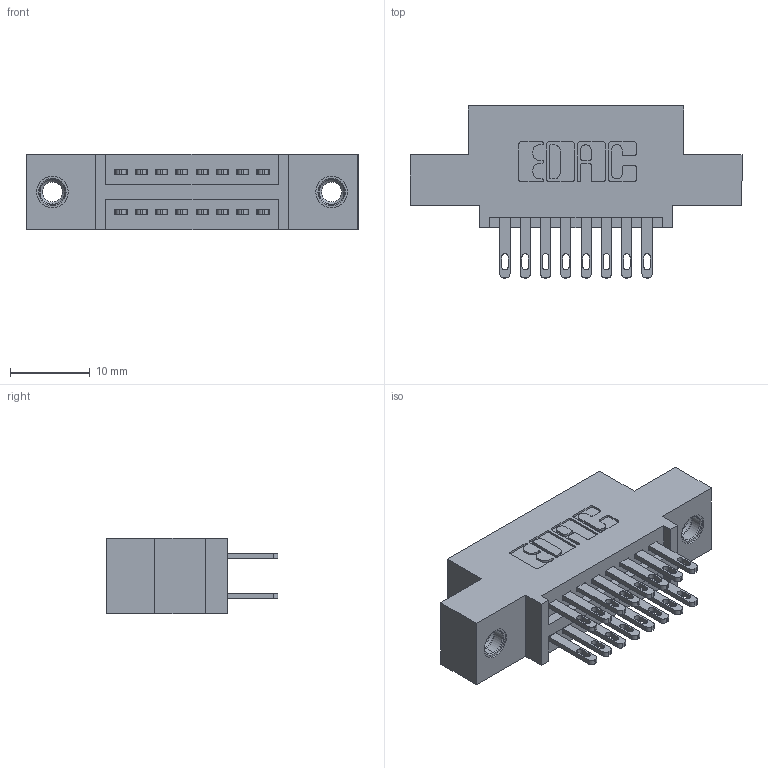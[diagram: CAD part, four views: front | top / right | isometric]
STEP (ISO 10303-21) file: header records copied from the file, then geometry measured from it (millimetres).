
FILE_DESCRIPTION (( 'STEP AP203' ), '1' );
FILE_NAME ('895-016-500-507.STEP', '2020-09-25T04:32:42', ( '' ), ( '' ), 'SwSTEP 2.0', 'SolidWorks 2020', '' );
FILE_SCHEMA (( 'CONFIG_CONTROL_DESIGN' ));
Length unit declared in the file: inch
Products named in the file (4): 845 Part_0.110 Offset - 0.156 Dia-TI; 345-250-001_345-250-005-103; 895-016-500-507; 345-292-001_345-293-100
Assembly tree (19 placements, depth 2):
  895-016-500-507
    845 Part_0.110 Offset - 0.156 Dia-TI
    345-292-001_345-293-100  x16
    345-250-001_345-250-005-103  x2
Bounding box: 41.53 x 21.51 x 9.4 mm (x, y, z)
Volume: 3680.6 mm3; surface area: 5065.9 mm2
Topology: 19 solids, 19 shells, 926 faces, 2745 edges, 1822 vertices
Faces by surface type: plane 548, cylinder 362, cone 12, torus 4
Entity records: 12102 total; most frequent: CARTESIAN_POINT 2043, ORIENTED_EDGE 1970, DIRECTION 1871, EDGE_CURVE 985, VECTOR 797, LINE 797, VERTEX_POINT 652, AXIS2_PLACEMENT_3D 537
